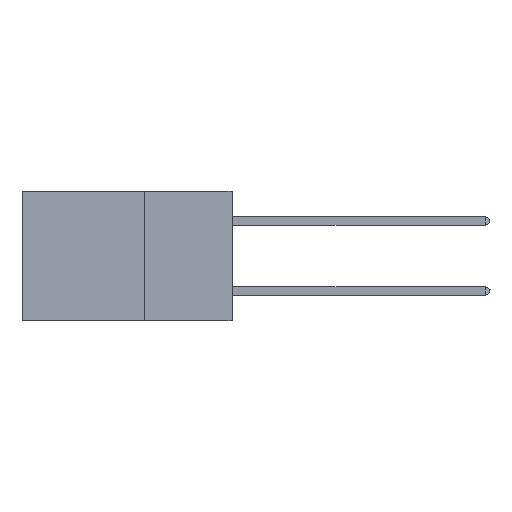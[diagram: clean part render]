
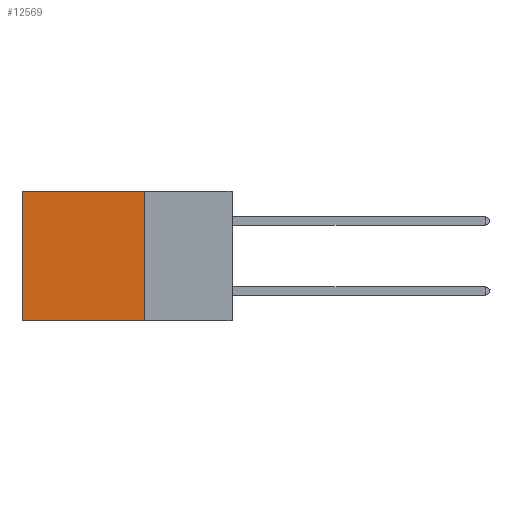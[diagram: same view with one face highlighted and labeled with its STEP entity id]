
A CAD part, left-side view. The second image highlights one B-rep face of the part: STEP entity #12569.
In plain terms, the highlighted planar face has unit normal (-1, 0, 0).
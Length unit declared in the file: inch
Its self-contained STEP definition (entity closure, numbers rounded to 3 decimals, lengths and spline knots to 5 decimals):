
#493 = CARTESIAN_POINT ( 'NONE',  ( 0.2875, 0.25, -0.37 ) ) ;
#1344 = CARTESIAN_POINT ( 'NONE',  ( 0.2875, 0.25, 0. ) ) ;
#1819 = CARTESIAN_POINT ( 'NONE',  ( 0.2875, 0.6, 0. ) ) ;
#1862 = VERTEX_POINT ( 'NONE', #18918 ) ;
#2316 = FACE_OUTER_BOUND ( 'NONE', #9833, .T. ) ;
#2611 = EDGE_CURVE ( 'NONE', #1862, #3644, #7326, .T. ) ;
#2839 = VERTEX_POINT ( 'NONE', #8093 ) ;
#3042 = DIRECTION ( 'NONE',  ( 0., 0., -1. ) ) ;
#3644 = VERTEX_POINT ( 'NONE', #3722 ) ;
#3712 = PLANE ( 'NONE',  #11602 ) ;
#3722 = CARTESIAN_POINT ( 'NONE',  ( 0.2875, 0.6, -0.37 ) ) ;
#3887 = VECTOR ( 'NONE', #13581, 39.37008 ) ;
#4193 = ORIENTED_EDGE ( 'NONE', *, *, #8138, .T. ) ;
#5022 = DIRECTION ( 'NONE',  ( 0., 1., 0. ) ) ;
#7326 = LINE ( 'NONE', #1819, #3887 ) ;
#8021 = EDGE_CURVE ( 'NONE', #15509, #2839, #15738, .T. ) ;
#8093 = CARTESIAN_POINT ( 'NONE',  ( 0.2875, 0.25, -0.37 ) ) ;
#8138 = EDGE_CURVE ( 'NONE', #15509, #1862, #10658, .T. ) ;
#8273 = EDGE_CURVE ( 'NONE', #2839, #3644, #17102, .T. ) ;
#9769 = ORIENTED_EDGE ( 'NONE', *, *, #2611, .T. ) ;
#9833 = EDGE_LOOP ( 'NONE', ( #9769, #12978, #16206, #4193 ) ) ;
#10658 = LINE ( 'NONE', #1344, #13624 ) ;
#11127 = VECTOR ( 'NONE', #5022, 39.37008 ) ;
#11364 = CARTESIAN_POINT ( 'NONE',  ( 0.2875, 0.25, 0. ) ) ;
#11602 = AXIS2_PLACEMENT_3D ( 'NONE', #14005, #15568, #17053 ) ;
#12569 = ADVANCED_FACE ( 'NONE', ( #2316 ), #3712, .F. ) ;
#12978 = ORIENTED_EDGE ( 'NONE', *, *, #8273, .F. ) ;
#13581 = DIRECTION ( 'NONE',  ( 0., 0., -1. ) ) ;
#13624 = VECTOR ( 'NONE', #18074, 39.37008 ) ;
#14005 = CARTESIAN_POINT ( 'NONE',  ( 0.2875, 0.25, 0. ) ) ;
#14576 = VECTOR ( 'NONE', #3042, 39.37008 ) ;
#15509 = VERTEX_POINT ( 'NONE', #11364 ) ;
#15568 = DIRECTION ( 'NONE',  ( 1., 0., 0. ) ) ;
#15738 = LINE ( 'NONE', #16309, #14576 ) ;
#16206 = ORIENTED_EDGE ( 'NONE', *, *, #8021, .F. ) ;
#16309 = CARTESIAN_POINT ( 'NONE',  ( 0.2875, 0.25, 0. ) ) ;
#17053 = DIRECTION ( 'NONE',  ( 0., 0., -1. ) ) ;
#17102 = LINE ( 'NONE', #493, #11127 ) ;
#18074 = DIRECTION ( 'NONE',  ( 0., 1., 0. ) ) ;
#18918 = CARTESIAN_POINT ( 'NONE',  ( 0.2875, 0.6, 0. ) ) ;
